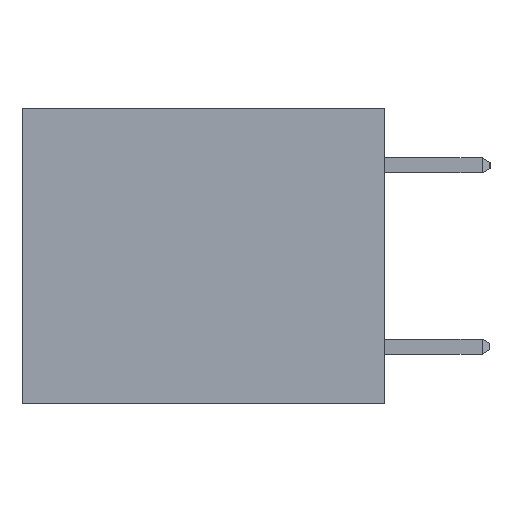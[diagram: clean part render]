
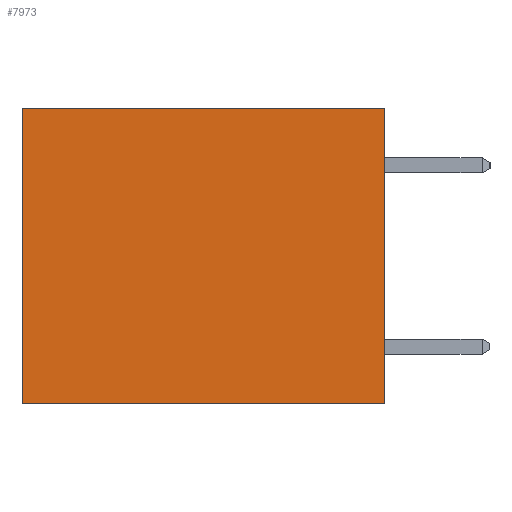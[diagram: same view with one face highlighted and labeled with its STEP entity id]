
A CAD part, left-side view. The second image highlights one B-rep face of the part: STEP entity #7973.
In plain terms, the highlighted planar face has unit normal (-1, 0, 0).
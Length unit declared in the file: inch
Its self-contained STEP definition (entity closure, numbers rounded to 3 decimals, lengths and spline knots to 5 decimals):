
#80 = CARTESIAN_POINT ( 'NONE',  ( 0.3165, 0., -0.49 ) ) ;
#1015 = ORIENTED_EDGE ( 'NONE', *, *, #4858, .T. ) ;
#1131 = ORIENTED_EDGE ( 'NONE', *, *, #1696, .F. ) ;
#1137 = LINE ( 'NONE', #5131, #15556 ) ;
#1321 = VECTOR ( 'NONE', #5911, 39.37008 ) ;
#1696 = EDGE_CURVE ( 'NONE', #4818, #8637, #13975, .T. ) ;
#2562 = VECTOR ( 'NONE', #12939, 39.37008 ) ;
#3702 = CARTESIAN_POINT ( 'NONE',  ( 0.3165, 0., -0.49 ) ) ;
#4092 = CARTESIAN_POINT ( 'NONE',  ( 0.3165, 0.6, 0. ) ) ;
#4818 = VERTEX_POINT ( 'NONE', #14272 ) ;
#4858 = EDGE_CURVE ( 'NONE', #12416, #8637, #5431, .T. ) ;
#5131 = CARTESIAN_POINT ( 'NONE',  ( 0.3165, 0., 0. ) ) ;
#5431 = LINE ( 'NONE', #7631, #2562 ) ;
#5911 = DIRECTION ( 'NONE',  ( 0., 0., -1. ) ) ;
#7037 = AXIS2_PLACEMENT_3D ( 'NONE', #3702, #12891, #7639 ) ;
#7631 = CARTESIAN_POINT ( 'NONE',  ( 0.3165, 0.6, -0.49 ) ) ;
#7639 = DIRECTION ( 'NONE',  ( 0., 0., -1. ) ) ;
#7670 = DIRECTION ( 'NONE',  ( 0., 1., 0. ) ) ;
#7973 = ADVANCED_FACE ( 'NONE', ( #15770 ), #16989, .F. ) ;
#8074 = DIRECTION ( 'NONE',  ( 0., 1., 0. ) ) ;
#8144 = VERTEX_POINT ( 'NONE', #14399 ) ;
#8382 = EDGE_CURVE ( 'NONE', #8144, #12416, #1137, .T. ) ;
#8637 = VERTEX_POINT ( 'NONE', #12333 ) ;
#9183 = EDGE_CURVE ( 'NONE', #8144, #4818, #12214, .T. ) ;
#10661 = ORIENTED_EDGE ( 'NONE', *, *, #9183, .F. ) ;
#12214 = LINE ( 'NONE', #12441, #1321 ) ;
#12333 = CARTESIAN_POINT ( 'NONE',  ( 0.3165, 0.6, -0.49 ) ) ;
#12416 = VERTEX_POINT ( 'NONE', #4092 ) ;
#12441 = CARTESIAN_POINT ( 'NONE',  ( 0.3165, 0., -0.49 ) ) ;
#12891 = DIRECTION ( 'NONE',  ( 1., 0., 0. ) ) ;
#12939 = DIRECTION ( 'NONE',  ( 0., 0., -1. ) ) ;
#13975 = LINE ( 'NONE', #80, #15822 ) ;
#14272 = CARTESIAN_POINT ( 'NONE',  ( 0.3165, 0., -0.49 ) ) ;
#14374 = ORIENTED_EDGE ( 'NONE', *, *, #8382, .T. ) ;
#14399 = CARTESIAN_POINT ( 'NONE',  ( 0.3165, 0., 0. ) ) ;
#15556 = VECTOR ( 'NONE', #7670, 39.37008 ) ;
#15770 = FACE_OUTER_BOUND ( 'NONE', #15799, .T. ) ;
#15799 = EDGE_LOOP ( 'NONE', ( #1015, #1131, #10661, #14374 ) ) ;
#15822 = VECTOR ( 'NONE', #8074, 39.37008 ) ;
#16989 = PLANE ( 'NONE',  #7037 ) ;
